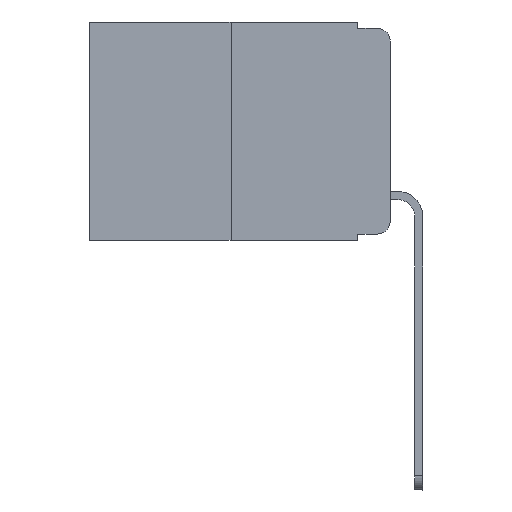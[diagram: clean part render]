
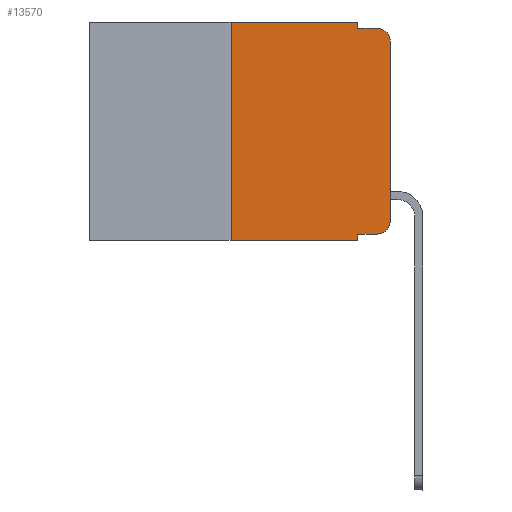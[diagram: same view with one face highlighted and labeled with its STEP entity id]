
A CAD part, left-side view. The second image highlights one B-rep face of the part: STEP entity #13570.
In plain terms, the highlighted planar face has unit normal (-1, 0, 0).
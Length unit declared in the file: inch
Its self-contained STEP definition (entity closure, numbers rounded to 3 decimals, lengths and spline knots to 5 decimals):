
#614 = VECTOR ( 'NONE', #16485, 39.37008 ) ;
#690 = LINE ( 'NONE', #10962, #10528 ) ;
#702 = LINE ( 'NONE', #13007, #7419 ) ;
#714 = LINE ( 'NONE', #11596, #3319 ) ;
#833 = EDGE_CURVE ( 'NONE', #9793, #14782, #690, .T. ) ;
#1162 = LINE ( 'NONE', #10463, #7797 ) ;
#1372 = ORIENTED_EDGE ( 'NONE', *, *, #8544, .T. ) ;
#1846 = DIRECTION ( 'NONE',  ( 0., 0., -1. ) ) ;
#2033 = DIRECTION ( 'NONE',  ( 0., 0., 1. ) ) ;
#2197 = CARTESIAN_POINT ( 'NONE',  ( 0., 0.02, -0.333 ) ) ;
#2283 = EDGE_CURVE ( 'NONE', #9680, #16342, #714, .T. ) ;
#2758 = CARTESIAN_POINT ( 'NONE',  ( 0., 0., -0.313 ) ) ;
#3263 = VECTOR ( 'NONE', #2033, 39.37008 ) ;
#3319 = VECTOR ( 'NONE', #6214, 39.37008 ) ;
#3400 = CARTESIAN_POINT ( 'NONE',  ( 0., 0.02, -0.313 ) ) ;
#3729 = ORIENTED_EDGE ( 'NONE', *, *, #7438, .F. ) ;
#3731 = VERTEX_POINT ( 'NONE', #16160 ) ;
#3732 = DIRECTION ( 'NONE',  ( 0., -1., 0. ) ) ;
#3893 = CARTESIAN_POINT ( 'NONE',  ( 0., 0.473, -0.343 ) ) ;
#3964 = ORIENTED_EDGE ( 'NONE', *, *, #2283, .F. ) ;
#3986 = AXIS2_PLACEMENT_3D ( 'NONE', #3400, #5799, #1846 ) ;
#4037 = CARTESIAN_POINT ( 'NONE',  ( 0., 0.051, 0. ) ) ;
#4206 = AXIS2_PLACEMENT_3D ( 'NONE', #8766, #7589, #12641 ) ;
#4584 = CARTESIAN_POINT ( 'NONE',  ( 0., 0.25, 0. ) ) ;
#4587 = EDGE_LOOP ( 'NONE', ( #1372, #5305, #11904, #3964, #7128, #3729, #8346, #7200, #10249, #9754 ) ) ;
#5305 = ORIENTED_EDGE ( 'NONE', *, *, #15335, .T. ) ;
#5799 = DIRECTION ( 'NONE',  ( -1., 0., 0. ) ) ;
#5916 = LINE ( 'NONE', #4584, #3263 ) ;
#6214 = DIRECTION ( 'NONE',  ( 0., 0., -1. ) ) ;
#6236 = CARTESIAN_POINT ( 'NONE',  ( 0., 0.02, -0.03 ) ) ;
#6275 = PLANE ( 'NONE',  #4206 ) ;
#6369 = CARTESIAN_POINT ( 'NONE',  ( 0., 0.051, -0.333 ) ) ;
#6852 = DIRECTION ( 'NONE',  ( 0., 0., -1. ) ) ;
#7052 = LINE ( 'NONE', #9788, #614 ) ;
#7091 = CARTESIAN_POINT ( 'NONE',  ( 0., 0.051, 0. ) ) ;
#7128 = ORIENTED_EDGE ( 'NONE', *, *, #7649, .F. ) ;
#7200 = ORIENTED_EDGE ( 'NONE', *, *, #7776, .F. ) ;
#7419 = VECTOR ( 'NONE', #10337, 39.37008 ) ;
#7438 = EDGE_CURVE ( 'NONE', #3731, #17081, #5916, .T. ) ;
#7589 = DIRECTION ( 'NONE',  ( 1., 0., 0. ) ) ;
#7649 = EDGE_CURVE ( 'NONE', #17081, #9680, #1162, .T. ) ;
#7776 = EDGE_CURVE ( 'NONE', #9793, #12155, #12254, .T. ) ;
#7797 = VECTOR ( 'NONE', #11633, 39.37008 ) ;
#8204 = AXIS2_PLACEMENT_3D ( 'NONE', #6236, #9144, #15723 ) ;
#8346 = ORIENTED_EDGE ( 'NONE', *, *, #8601, .T. ) ;
#8411 = CARTESIAN_POINT ( 'NONE',  ( 0., 0.051, -0.343 ) ) ;
#8544 = EDGE_CURVE ( 'NONE', #13870, #10298, #702, .T. ) ;
#8566 = VECTOR ( 'NONE', #3732, 39.37008 ) ;
#8601 = EDGE_CURVE ( 'NONE', #3731, #12155, #17386, .T. ) ;
#8766 = CARTESIAN_POINT ( 'NONE',  ( 0., 0.473, 0. ) ) ;
#9144 = DIRECTION ( 'NONE',  ( -1., 0., 0. ) ) ;
#9213 = VECTOR ( 'NONE', #6852, 39.37008 ) ;
#9360 = CARTESIAN_POINT ( 'NONE',  ( 0., 0., -0.03 ) ) ;
#9614 = CIRCLE ( 'NONE', #8204, 0.02 ) ;
#9680 = VERTEX_POINT ( 'NONE', #7091 ) ;
#9732 = CARTESIAN_POINT ( 'NONE',  ( 0., 0.25, 0. ) ) ;
#9754 = ORIENTED_EDGE ( 'NONE', *, *, #15516, .T. ) ;
#9788 = CARTESIAN_POINT ( 'NONE',  ( 0., 0.051, -0.01 ) ) ;
#9793 = VERTEX_POINT ( 'NONE', #6369 ) ;
#10249 = ORIENTED_EDGE ( 'NONE', *, *, #833, .T. ) ;
#10298 = VERTEX_POINT ( 'NONE', #9360 ) ;
#10337 = DIRECTION ( 'NONE',  ( 0., 0., 1. ) ) ;
#10463 = CARTESIAN_POINT ( 'NONE',  ( 0., 0.473, 0. ) ) ;
#10528 = VECTOR ( 'NONE', #11060, 39.37008 ) ;
#10962 = CARTESIAN_POINT ( 'NONE',  ( 0., 0.051, -0.333 ) ) ;
#11060 = DIRECTION ( 'NONE',  ( 0., -1., 0. ) ) ;
#11596 = CARTESIAN_POINT ( 'NONE',  ( 0., 0.051, 0. ) ) ;
#11633 = DIRECTION ( 'NONE',  ( 0., -1., 0. ) ) ;
#11904 = ORIENTED_EDGE ( 'NONE', *, *, #14605, .F. ) ;
#12155 = VERTEX_POINT ( 'NONE', #8411 ) ;
#12254 = LINE ( 'NONE', #4037, #9213 ) ;
#12606 = CARTESIAN_POINT ( 'NONE',  ( 0., 0.051, -0.01 ) ) ;
#12641 = DIRECTION ( 'NONE',  ( 0., 0., -1. ) ) ;
#13007 = CARTESIAN_POINT ( 'NONE',  ( 0., 0., 0. ) ) ;
#13570 = ADVANCED_FACE ( 'NONE', ( #15425 ), #6275, .F. ) ;
#13870 = VERTEX_POINT ( 'NONE', #2758 ) ;
#14466 = VERTEX_POINT ( 'NONE', #14540 ) ;
#14540 = CARTESIAN_POINT ( 'NONE',  ( 0., 0.02, -0.01 ) ) ;
#14605 = EDGE_CURVE ( 'NONE', #16342, #14466, #7052, .T. ) ;
#14782 = VERTEX_POINT ( 'NONE', #2197 ) ;
#15315 = CIRCLE ( 'NONE', #3986, 0.02 ) ;
#15335 = EDGE_CURVE ( 'NONE', #10298, #14466, #9614, .T. ) ;
#15425 = FACE_OUTER_BOUND ( 'NONE', #4587, .T. ) ;
#15516 = EDGE_CURVE ( 'NONE', #14782, #13870, #15315, .T. ) ;
#15723 = DIRECTION ( 'NONE',  ( 0., 0., -1. ) ) ;
#16160 = CARTESIAN_POINT ( 'NONE',  ( 0., 0.25, -0.343 ) ) ;
#16342 = VERTEX_POINT ( 'NONE', #12606 ) ;
#16485 = DIRECTION ( 'NONE',  ( 0., -1., 0. ) ) ;
#17081 = VERTEX_POINT ( 'NONE', #9732 ) ;
#17386 = LINE ( 'NONE', #3893, #8566 ) ;
